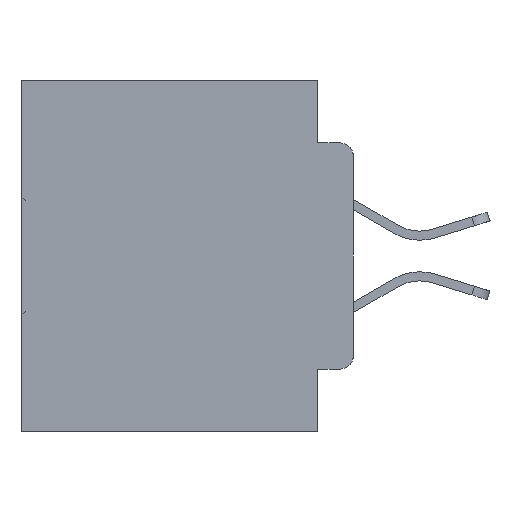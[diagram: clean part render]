
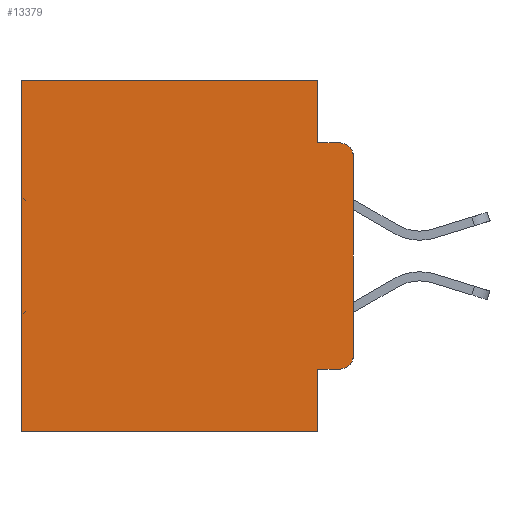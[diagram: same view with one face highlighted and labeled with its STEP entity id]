
A CAD part, left-side view. The second image highlights one B-rep face of the part: STEP entity #13379.
In plain terms, the highlighted planar face has unit normal (-1, 0, 0).
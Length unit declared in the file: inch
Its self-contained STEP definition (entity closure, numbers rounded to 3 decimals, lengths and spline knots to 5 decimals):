
#39 = CARTESIAN_POINT ( 'NONE',  ( 0.298, 0.473, 0. ) ) ;
#526 = CARTESIAN_POINT ( 'NONE',  ( 0.298, 0.473, -0.5 ) ) ;
#1278 = VERTEX_POINT ( 'NONE', #11556 ) ;
#1846 = ORIENTED_EDGE ( 'NONE', *, *, #18717, .T. ) ;
#2097 = CARTESIAN_POINT ( 'NONE',  ( 0.298, 0., 0. ) ) ;
#2735 = CARTESIAN_POINT ( 'NONE',  ( 0.298, 0.051, -0.5 ) ) ;
#2842 = EDGE_LOOP ( 'NONE', ( #27766, #1846, #14213, #22885, #6886, #34180, #34079, #25948, #13122, #9811 ) ) ;
#3159 = CARTESIAN_POINT ( 'NONE',  ( 0.298, 0.051, 0. ) ) ;
#3285 = VERTEX_POINT ( 'NONE', #18675 ) ;
#3921 = DIRECTION ( 'NONE',  ( -1., 0., 0. ) ) ;
#4192 = CARTESIAN_POINT ( 'NONE',  ( 0.298, 0.051, -0.4115 ) ) ;
#4218 = EDGE_CURVE ( 'NONE', #3285, #20978, #9250, .T. ) ;
#4806 = DIRECTION ( 'NONE',  ( 1., 0., 0. ) ) ;
#5024 = VERTEX_POINT ( 'NONE', #4192 ) ;
#5330 = EDGE_CURVE ( 'NONE', #1278, #10130, #29130, .T. ) ;
#6057 = LINE ( 'NONE', #9235, #26573 ) ;
#6846 = VERTEX_POINT ( 'NONE', #2735 ) ;
#6886 = ORIENTED_EDGE ( 'NONE', *, *, #26064, .T. ) ;
#6941 = LINE ( 'NONE', #3159, #20448 ) ;
#6989 = VERTEX_POINT ( 'NONE', #23789 ) ;
#7792 = CARTESIAN_POINT ( 'NONE',  ( 0.298, 0.051, -0.0885 ) ) ;
#8125 = AXIS2_PLACEMENT_3D ( 'NONE', #20112, #3921, #22728 ) ;
#8308 = VERTEX_POINT ( 'NONE', #32394 ) ;
#8572 = LINE ( 'NONE', #27921, #28962 ) ;
#9235 = CARTESIAN_POINT ( 'NONE',  ( 0.298, 0.051, -0.4115 ) ) ;
#9250 = LINE ( 'NONE', #23181, #14801 ) ;
#9811 = ORIENTED_EDGE ( 'NONE', *, *, #12216, .T. ) ;
#10130 = VERTEX_POINT ( 'NONE', #10508 ) ;
#10508 = CARTESIAN_POINT ( 'NONE',  ( 0.298, 0., -0.3915 ) ) ;
#10837 = VECTOR ( 'NONE', #18090, 39.37008 ) ;
#11531 = EDGE_CURVE ( 'NONE', #20978, #28640, #21908, .T. ) ;
#11556 = CARTESIAN_POINT ( 'NONE',  ( 0.298, 0., -0.1085 ) ) ;
#11696 = LINE ( 'NONE', #15436, #10837 ) ;
#12014 = CARTESIAN_POINT ( 'NONE',  ( 0.298, 0.051, -0.0885 ) ) ;
#12216 = EDGE_CURVE ( 'NONE', #6989, #10130, #14427, .T. ) ;
#12435 = VERTEX_POINT ( 'NONE', #526 ) ;
#13107 = CARTESIAN_POINT ( 'NONE',  ( 0.298, 0.02, -0.3915 ) ) ;
#13122 = ORIENTED_EDGE ( 'NONE', *, *, #19408, .T. ) ;
#13379 = ADVANCED_FACE ( 'NONE', ( #14758 ), #18293, .F. ) ;
#14213 = ORIENTED_EDGE ( 'NONE', *, *, #11531, .F. ) ;
#14301 = VECTOR ( 'NONE', #15180, 39.37008 ) ;
#14427 = CIRCLE ( 'NONE', #24563, 0.02 ) ;
#14758 = FACE_OUTER_BOUND ( 'NONE', #2842, .T. ) ;
#14801 = VECTOR ( 'NONE', #15038, 39.37008 ) ;
#15038 = DIRECTION ( 'NONE',  ( 0., 0., -1. ) ) ;
#15180 = DIRECTION ( 'NONE',  ( 0., 0., -1. ) ) ;
#15436 = CARTESIAN_POINT ( 'NONE',  ( 0.298, 0., 0. ) ) ;
#15803 = DIRECTION ( 'NONE',  ( 0., 0., -1. ) ) ;
#17415 = LINE ( 'NONE', #39, #23608 ) ;
#18090 = DIRECTION ( 'NONE',  ( 0., 1., 0. ) ) ;
#18293 = PLANE ( 'NONE',  #18409 ) ;
#18409 = AXIS2_PLACEMENT_3D ( 'NONE', #2097, #4806, #23592 ) ;
#18636 = DIRECTION ( 'NONE',  ( 0., -1., 0. ) ) ;
#18675 = CARTESIAN_POINT ( 'NONE',  ( 0.298, 0.051, 0. ) ) ;
#18717 = EDGE_CURVE ( 'NONE', #1278, #28640, #24553, .T. ) ;
#18939 = DIRECTION ( 'NONE',  ( 0., 0., -1. ) ) ;
#19408 = EDGE_CURVE ( 'NONE', #5024, #6989, #6057, .T. ) ;
#20112 = CARTESIAN_POINT ( 'NONE',  ( 0.298, 0.02, -0.1085 ) ) ;
#20283 = VECTOR ( 'NONE', #18636, 39.37008 ) ;
#20448 = VECTOR ( 'NONE', #21996, 39.37008 ) ;
#20978 = VERTEX_POINT ( 'NONE', #12014 ) ;
#21087 = CARTESIAN_POINT ( 'NONE',  ( 0.298, 0.02, -0.0885 ) ) ;
#21908 = LINE ( 'NONE', #7792, #20283 ) ;
#21996 = DIRECTION ( 'NONE',  ( 0., 0., -1. ) ) ;
#22728 = DIRECTION ( 'NONE',  ( 0., 0., -1. ) ) ;
#22885 = ORIENTED_EDGE ( 'NONE', *, *, #4218, .F. ) ;
#23181 = CARTESIAN_POINT ( 'NONE',  ( 0.298, 0.051, 0. ) ) ;
#23592 = DIRECTION ( 'NONE',  ( 0., 0., -1. ) ) ;
#23608 = VECTOR ( 'NONE', #18939, 39.37008 ) ;
#23789 = CARTESIAN_POINT ( 'NONE',  ( 0.298, 0.02, -0.4115 ) ) ;
#24553 = CIRCLE ( 'NONE', #8125, 0.02 ) ;
#24563 = AXIS2_PLACEMENT_3D ( 'NONE', #13107, #31549, #15803 ) ;
#25948 = ORIENTED_EDGE ( 'NONE', *, *, #26416, .F. ) ;
#26064 = EDGE_CURVE ( 'NONE', #3285, #8308, #11696, .T. ) ;
#26416 = EDGE_CURVE ( 'NONE', #5024, #6846, #6941, .T. ) ;
#26573 = VECTOR ( 'NONE', #27866, 39.37008 ) ;
#27766 = ORIENTED_EDGE ( 'NONE', *, *, #5330, .F. ) ;
#27866 = DIRECTION ( 'NONE',  ( 0., -1., 0. ) ) ;
#27921 = CARTESIAN_POINT ( 'NONE',  ( 0.298, 0., -0.5 ) ) ;
#28097 = CARTESIAN_POINT ( 'NONE',  ( 0.298, 0., 0. ) ) ;
#28640 = VERTEX_POINT ( 'NONE', #21087 ) ;
#28962 = VECTOR ( 'NONE', #30552, 39.37008 ) ;
#29130 = LINE ( 'NONE', #28097, #14301 ) ;
#29526 = EDGE_CURVE ( 'NONE', #6846, #12435, #8572, .T. ) ;
#29932 = EDGE_CURVE ( 'NONE', #8308, #12435, #17415, .T. ) ;
#30552 = DIRECTION ( 'NONE',  ( 0., 1., 0. ) ) ;
#31549 = DIRECTION ( 'NONE',  ( -1., 0., 0. ) ) ;
#32394 = CARTESIAN_POINT ( 'NONE',  ( 0.298, 0.473, 0. ) ) ;
#34079 = ORIENTED_EDGE ( 'NONE', *, *, #29526, .F. ) ;
#34180 = ORIENTED_EDGE ( 'NONE', *, *, #29932, .T. ) ;
